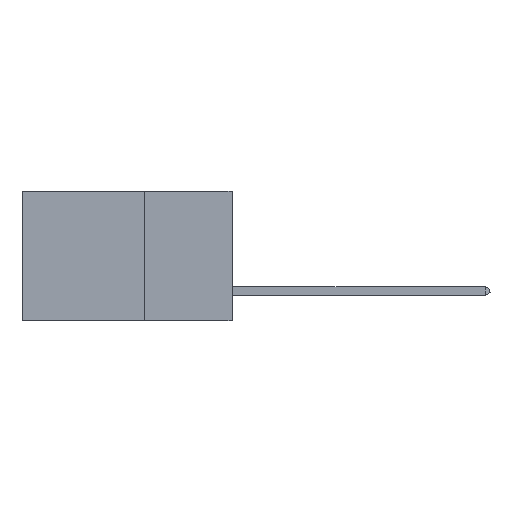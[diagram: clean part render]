
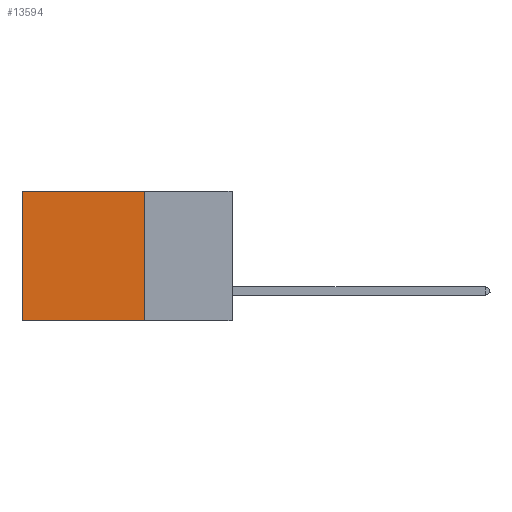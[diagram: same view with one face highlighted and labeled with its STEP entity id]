
A CAD part, left-side view. The second image highlights one B-rep face of the part: STEP entity #13594.
In plain terms, the highlighted planar face has unit normal (-1, 0, 0).
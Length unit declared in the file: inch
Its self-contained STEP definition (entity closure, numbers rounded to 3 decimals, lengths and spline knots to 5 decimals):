
#109 = CARTESIAN_POINT ( 'NONE',  ( 0.2875, 0.6, 0. ) ) ;
#232 = VECTOR ( 'NONE', #8324, 39.37008 ) ;
#863 = LINE ( 'NONE', #5936, #14438 ) ;
#1030 = EDGE_LOOP ( 'NONE', ( #20464, #2489, #1762, #21018 ) ) ;
#1240 = VERTEX_POINT ( 'NONE', #9954 ) ;
#1335 = PLANE ( 'NONE',  #2828 ) ;
#1762 = ORIENTED_EDGE ( 'NONE', *, *, #2835, .F. ) ;
#2340 = FACE_OUTER_BOUND ( 'NONE', #1030, .T. ) ;
#2489 = ORIENTED_EDGE ( 'NONE', *, *, #10945, .F. ) ;
#2828 = AXIS2_PLACEMENT_3D ( 'NONE', #8049, #13234, #16788 ) ;
#2835 = EDGE_CURVE ( 'NONE', #1240, #3503, #863, .T. ) ;
#3393 = EDGE_CURVE ( 'NONE', #1240, #14399, #8236, .T. ) ;
#3503 = VERTEX_POINT ( 'NONE', #10832 ) ;
#3521 = CARTESIAN_POINT ( 'NONE',  ( 0.2875, 0.25, 0. ) ) ;
#5497 = LINE ( 'NONE', #109, #232 ) ;
#5936 = CARTESIAN_POINT ( 'NONE',  ( 0.2875, 0.25, 0. ) ) ;
#7336 = CARTESIAN_POINT ( 'NONE',  ( 0.2875, 0.25, -0.37 ) ) ;
#8049 = CARTESIAN_POINT ( 'NONE',  ( 0.2875, 0.25, 0. ) ) ;
#8236 = LINE ( 'NONE', #3521, #8480 ) ;
#8324 = DIRECTION ( 'NONE',  ( 0., 0., -1. ) ) ;
#8480 = VECTOR ( 'NONE', #8735, 39.37008 ) ;
#8735 = DIRECTION ( 'NONE',  ( 0., 1., 0. ) ) ;
#9481 = EDGE_CURVE ( 'NONE', #14399, #18606, #5497, .T. ) ;
#9578 = DIRECTION ( 'NONE',  ( 0., 0., -1. ) ) ;
#9954 = CARTESIAN_POINT ( 'NONE',  ( 0.2875, 0.25, 0. ) ) ;
#10832 = CARTESIAN_POINT ( 'NONE',  ( 0.2875, 0.25, -0.37 ) ) ;
#10945 = EDGE_CURVE ( 'NONE', #3503, #18606, #11031, .T. ) ;
#11031 = LINE ( 'NONE', #7336, #17726 ) ;
#13234 = DIRECTION ( 'NONE',  ( 1., 0., 0. ) ) ;
#13594 = ADVANCED_FACE ( 'NONE', ( #2340 ), #1335, .F. ) ;
#14169 = CARTESIAN_POINT ( 'NONE',  ( 0.2875, 0.6, -0.37 ) ) ;
#14399 = VERTEX_POINT ( 'NONE', #15102 ) ;
#14438 = VECTOR ( 'NONE', #9578, 39.37008 ) ;
#15102 = CARTESIAN_POINT ( 'NONE',  ( 0.2875, 0.6, 0. ) ) ;
#16788 = DIRECTION ( 'NONE',  ( 0., 0., -1. ) ) ;
#17726 = VECTOR ( 'NONE', #21091, 39.37008 ) ;
#18606 = VERTEX_POINT ( 'NONE', #14169 ) ;
#20464 = ORIENTED_EDGE ( 'NONE', *, *, #9481, .T. ) ;
#21018 = ORIENTED_EDGE ( 'NONE', *, *, #3393, .T. ) ;
#21091 = DIRECTION ( 'NONE',  ( 0., 1., 0. ) ) ;
